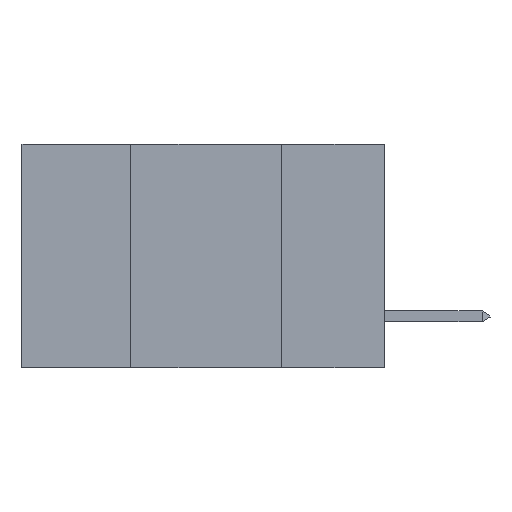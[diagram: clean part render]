
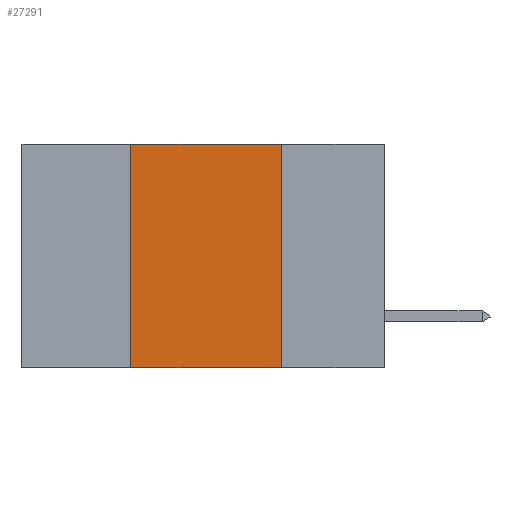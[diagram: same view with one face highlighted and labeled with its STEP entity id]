
A CAD part, left-side view. The second image highlights one B-rep face of the part: STEP entity #27291.
In plain terms, the highlighted planar face has unit normal (-1, 0, 0).
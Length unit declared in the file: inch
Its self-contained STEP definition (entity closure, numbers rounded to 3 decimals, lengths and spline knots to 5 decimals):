
#252 = AXIS2_PLACEMENT_3D ( 'NONE', #13339, #24446, #35925 ) ;
#1243 = CARTESIAN_POINT ( 'NONE',  ( 0., 0.17, 0. ) ) ;
#1987 = CARTESIAN_POINT ( 'NONE',  ( 0., 0.42, -0.37 ) ) ;
#2090 = VERTEX_POINT ( 'NONE', #42241 ) ;
#2661 = CARTESIAN_POINT ( 'NONE',  ( 0., 0.42, 0. ) ) ;
#3290 = LINE ( 'NONE', #39639, #45992 ) ;
#4595 = ORIENTED_EDGE ( 'NONE', *, *, #5485, .F. ) ;
#5485 = EDGE_CURVE ( 'NONE', #11441, #2090, #12059, .T. ) ;
#5671 = DIRECTION ( 'NONE',  ( 0., -1., 0. ) ) ;
#7317 = VERTEX_POINT ( 'NONE', #42876 ) ;
#7879 = EDGE_LOOP ( 'NONE', ( #41864, #44007, #4595, #21591 ) ) ;
#11441 = VERTEX_POINT ( 'NONE', #1987 ) ;
#11913 = DIRECTION ( 'NONE',  ( 0., 0., -1. ) ) ;
#12059 = LINE ( 'NONE', #2661, #22394 ) ;
#13339 = CARTESIAN_POINT ( 'NONE',  ( 0., 0.6, 0. ) ) ;
#14244 = LINE ( 'NONE', #31595, #17122 ) ;
#16650 = PLANE ( 'NONE',  #252 ) ;
#17122 = VECTOR ( 'NONE', #11913, 39.37008 ) ;
#19675 = VERTEX_POINT ( 'NONE', #1243 ) ;
#21591 = ORIENTED_EDGE ( 'NONE', *, *, #26037, .T. ) ;
#21808 = LINE ( 'NONE', #37264, #25461 ) ;
#22394 = VECTOR ( 'NONE', #27379, 39.37008 ) ;
#24446 = DIRECTION ( 'NONE',  ( 1., 0., 0. ) ) ;
#25461 = VECTOR ( 'NONE', #48125, 39.37008 ) ;
#26037 = EDGE_CURVE ( 'NONE', #11441, #7317, #3290, .T. ) ;
#27291 = ADVANCED_FACE ( 'NONE', ( #40374 ), #16650, .F. ) ;
#27379 = DIRECTION ( 'NONE',  ( 0., 0., 1. ) ) ;
#31595 = CARTESIAN_POINT ( 'NONE',  ( 0., 0.17, 0. ) ) ;
#35925 = DIRECTION ( 'NONE',  ( 0., 0., -1. ) ) ;
#37264 = CARTESIAN_POINT ( 'NONE',  ( 0., 0.6, 0. ) ) ;
#38499 = EDGE_CURVE ( 'NONE', #2090, #19675, #21808, .T. ) ;
#39639 = CARTESIAN_POINT ( 'NONE',  ( 0., 0.6, -0.37 ) ) ;
#40374 = FACE_OUTER_BOUND ( 'NONE', #7879, .T. ) ;
#41864 = ORIENTED_EDGE ( 'NONE', *, *, #42377, .F. ) ;
#42241 = CARTESIAN_POINT ( 'NONE',  ( 0., 0.42, 0. ) ) ;
#42377 = EDGE_CURVE ( 'NONE', #19675, #7317, #14244, .T. ) ;
#42876 = CARTESIAN_POINT ( 'NONE',  ( 0., 0.17, -0.37 ) ) ;
#44007 = ORIENTED_EDGE ( 'NONE', *, *, #38499, .F. ) ;
#45992 = VECTOR ( 'NONE', #5671, 39.37008 ) ;
#48125 = DIRECTION ( 'NONE',  ( 0., -1., 0. ) ) ;
